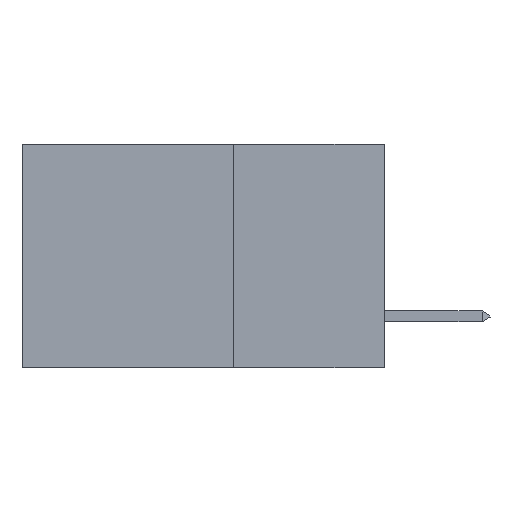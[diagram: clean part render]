
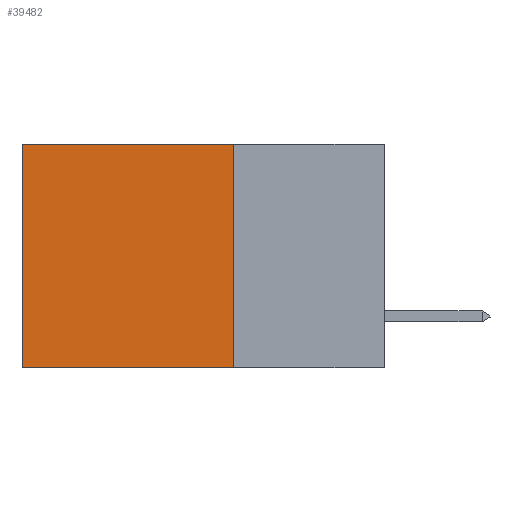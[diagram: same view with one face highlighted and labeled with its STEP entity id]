
A CAD part, left-side view. The second image highlights one B-rep face of the part: STEP entity #39482.
In plain terms, the highlighted planar face has unit normal (-1, 0, 0).
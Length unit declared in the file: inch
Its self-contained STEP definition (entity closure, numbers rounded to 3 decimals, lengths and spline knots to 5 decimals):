
#833 = DIRECTION ( 'NONE',  ( 0., 0., -1. ) ) ;
#2753 = LINE ( 'NONE', #46658, #28304 ) ;
#3781 = EDGE_CURVE ( 'NONE', #47827, #37049, #2753, .T. ) ;
#4594 = CARTESIAN_POINT ( 'NONE',  ( 0.2875, 0.25, 0. ) ) ;
#7628 = DIRECTION ( 'NONE',  ( 0., 0., -1. ) ) ;
#8719 = DIRECTION ( 'NONE',  ( 0., 1., 0. ) ) ;
#9272 = ORIENTED_EDGE ( 'NONE', *, *, #3781, .T. ) ;
#9458 = LINE ( 'NONE', #40547, #42063 ) ;
#10262 = CARTESIAN_POINT ( 'NONE',  ( 0.2875, 0.6, 0. ) ) ;
#10394 = DIRECTION ( 'NONE',  ( 0., 1., 0. ) ) ;
#15299 = LINE ( 'NONE', #4594, #23641 ) ;
#16303 = ORIENTED_EDGE ( 'NONE', *, *, #18809, .F. ) ;
#16911 = ORIENTED_EDGE ( 'NONE', *, *, #26468, .T. ) ;
#18809 = EDGE_CURVE ( 'NONE', #47160, #38228, #9458, .T. ) ;
#21834 = CARTESIAN_POINT ( 'NONE',  ( 0.2875, 0.25, -0.37 ) ) ;
#22492 = CARTESIAN_POINT ( 'NONE',  ( 0.2875, 0.6, -0.37 ) ) ;
#22875 = DIRECTION ( 'NONE',  ( 1., 0., 0. ) ) ;
#23641 = VECTOR ( 'NONE', #38748, 39.37008 ) ;
#26430 = CARTESIAN_POINT ( 'NONE',  ( 0.2875, 0.25, 0. ) ) ;
#26468 = EDGE_CURVE ( 'NONE', #37049, #38228, #37283, .T. ) ;
#26553 = PLANE ( 'NONE',  #32504 ) ;
#26932 = EDGE_CURVE ( 'NONE', #47827, #47160, #15299, .T. ) ;
#28304 = VECTOR ( 'NONE', #8719, 39.37008 ) ;
#32504 = AXIS2_PLACEMENT_3D ( 'NONE', #45398, #22875, #7628 ) ;
#34583 = EDGE_LOOP ( 'NONE', ( #16911, #16303, #36935, #9272 ) ) ;
#36935 = ORIENTED_EDGE ( 'NONE', *, *, #26932, .F. ) ;
#37049 = VERTEX_POINT ( 'NONE', #10262 ) ;
#37283 = LINE ( 'NONE', #42456, #38459 ) ;
#38228 = VERTEX_POINT ( 'NONE', #22492 ) ;
#38459 = VECTOR ( 'NONE', #833, 39.37008 ) ;
#38748 = DIRECTION ( 'NONE',  ( 0., 0., -1. ) ) ;
#39231 = FACE_OUTER_BOUND ( 'NONE', #34583, .T. ) ;
#39482 = ADVANCED_FACE ( 'NONE', ( #39231 ), #26553, .F. ) ;
#40547 = CARTESIAN_POINT ( 'NONE',  ( 0.2875, 0.25, -0.37 ) ) ;
#42063 = VECTOR ( 'NONE', #10394, 39.37008 ) ;
#42456 = CARTESIAN_POINT ( 'NONE',  ( 0.2875, 0.6, 0. ) ) ;
#45398 = CARTESIAN_POINT ( 'NONE',  ( 0.2875, 0.25, 0. ) ) ;
#46658 = CARTESIAN_POINT ( 'NONE',  ( 0.2875, 0.25, 0. ) ) ;
#47160 = VERTEX_POINT ( 'NONE', #21834 ) ;
#47827 = VERTEX_POINT ( 'NONE', #26430 ) ;
